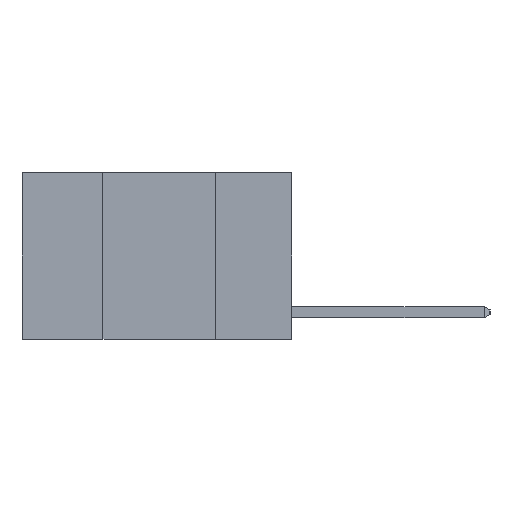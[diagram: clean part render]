
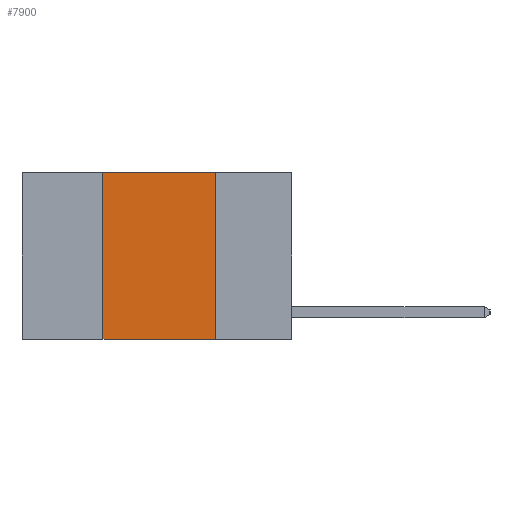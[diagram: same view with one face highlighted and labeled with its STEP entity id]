
A CAD part, left-side view. The second image highlights one B-rep face of the part: STEP entity #7900.
In plain terms, the highlighted planar face has unit normal (-1, 0, 0).
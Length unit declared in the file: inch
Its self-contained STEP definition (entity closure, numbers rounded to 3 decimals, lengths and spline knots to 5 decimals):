
#322 = DIRECTION ( 'NONE',  ( 0., 0., -1. ) ) ;
#545 = EDGE_CURVE ( 'NONE', #8220, #8987, #3503, .T. ) ;
#609 = VERTEX_POINT ( 'NONE', #5657 ) ;
#1026 = AXIS2_PLACEMENT_3D ( 'NONE', #4630, #5486, #322 ) ;
#1215 = CARTESIAN_POINT ( 'NONE',  ( 0., 0.17, -0.37 ) ) ;
#1503 = VECTOR ( 'NONE', #7340, 39.37008 ) ;
#2692 = DIRECTION ( 'NONE',  ( 0., 0., -1. ) ) ;
#3208 = FACE_OUTER_BOUND ( 'NONE', #11050, .T. ) ;
#3445 = EDGE_CURVE ( 'NONE', #609, #5370, #5074, .T. ) ;
#3452 = ORIENTED_EDGE ( 'NONE', *, *, #3445, .F. ) ;
#3476 = EDGE_CURVE ( 'NONE', #5370, #8987, #4790, .T. ) ;
#3482 = CARTESIAN_POINT ( 'NONE',  ( 0., 0.17, 0. ) ) ;
#3483 = DIRECTION ( 'NONE',  ( 0., -1., 0. ) ) ;
#3503 = LINE ( 'NONE', #6696, #1503 ) ;
#3996 = ORIENTED_EDGE ( 'NONE', *, *, #4655, .F. ) ;
#4630 = CARTESIAN_POINT ( 'NONE',  ( 0., 0.6, 0. ) ) ;
#4655 = EDGE_CURVE ( 'NONE', #8220, #609, #8922, .T. ) ;
#4790 = LINE ( 'NONE', #9570, #6810 ) ;
#5074 = LINE ( 'NONE', #7791, #9352 ) ;
#5370 = VERTEX_POINT ( 'NONE', #3482 ) ;
#5486 = DIRECTION ( 'NONE',  ( 1., 0., 0. ) ) ;
#5657 = CARTESIAN_POINT ( 'NONE',  ( 0., 0.42, 0. ) ) ;
#6390 = VECTOR ( 'NONE', #11122, 39.37008 ) ;
#6696 = CARTESIAN_POINT ( 'NONE',  ( 0., 0.6, -0.37 ) ) ;
#6810 = VECTOR ( 'NONE', #2692, 39.37008 ) ;
#7340 = DIRECTION ( 'NONE',  ( 0., -1., 0. ) ) ;
#7561 = ORIENTED_EDGE ( 'NONE', *, *, #3476, .F. ) ;
#7590 = CARTESIAN_POINT ( 'NONE',  ( 0., 0.42, -0.37 ) ) ;
#7791 = CARTESIAN_POINT ( 'NONE',  ( 0., 0.6, 0. ) ) ;
#7900 = ADVANCED_FACE ( 'NONE', ( #3208 ), #9750, .F. ) ;
#8220 = VERTEX_POINT ( 'NONE', #7590 ) ;
#8922 = LINE ( 'NONE', #10256, #6390 ) ;
#8987 = VERTEX_POINT ( 'NONE', #1215 ) ;
#9352 = VECTOR ( 'NONE', #3483, 39.37008 ) ;
#9427 = ORIENTED_EDGE ( 'NONE', *, *, #545, .T. ) ;
#9570 = CARTESIAN_POINT ( 'NONE',  ( 0., 0.17, 0. ) ) ;
#9750 = PLANE ( 'NONE',  #1026 ) ;
#10256 = CARTESIAN_POINT ( 'NONE',  ( 0., 0.42, 0. ) ) ;
#11050 = EDGE_LOOP ( 'NONE', ( #7561, #3452, #3996, #9427 ) ) ;
#11122 = DIRECTION ( 'NONE',  ( 0., 0., 1. ) ) ;
